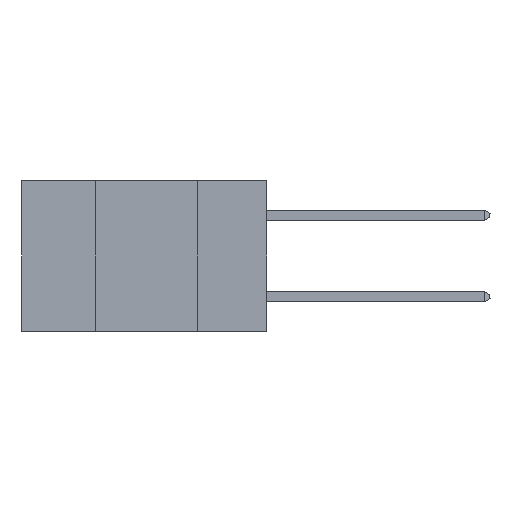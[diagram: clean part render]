
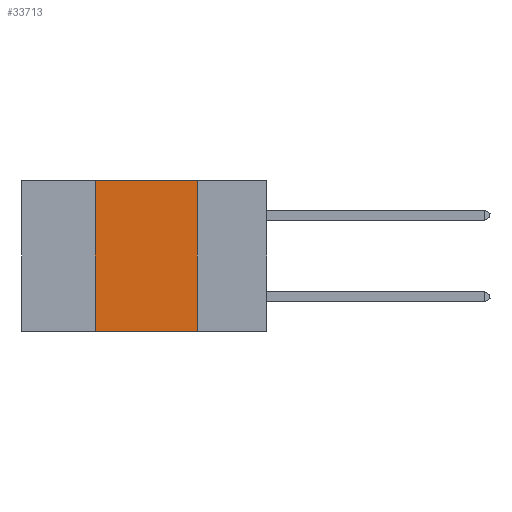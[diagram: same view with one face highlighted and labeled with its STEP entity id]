
A CAD part, left-side view. The second image highlights one B-rep face of the part: STEP entity #33713.
In plain terms, the highlighted planar face has unit normal (-1, 0, 0).
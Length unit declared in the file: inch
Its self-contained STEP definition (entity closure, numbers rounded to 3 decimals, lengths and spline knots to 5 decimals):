
#1861 = AXIS2_PLACEMENT_3D ( 'NONE', #5894, #24142, #1990 ) ;
#1990 = DIRECTION ( 'NONE',  ( 0., 0., -1. ) ) ;
#2196 = CARTESIAN_POINT ( 'NONE',  ( 0., 0.17, 0. ) ) ;
#4526 = VECTOR ( 'NONE', #17245, 39.37008 ) ;
#4668 = CARTESIAN_POINT ( 'NONE',  ( 0., 0.6, -0.37 ) ) ;
#4894 = EDGE_CURVE ( 'NONE', #17789, #32088, #27864, .T. ) ;
#5894 = CARTESIAN_POINT ( 'NONE',  ( 0., 0.6, 0. ) ) ;
#7902 = LINE ( 'NONE', #2196, #39862 ) ;
#8974 = ORIENTED_EDGE ( 'NONE', *, *, #31294, .F. ) ;
#9888 = DIRECTION ( 'NONE',  ( 0., 0., -1. ) ) ;
#9952 = FACE_OUTER_BOUND ( 'NONE', #28136, .T. ) ;
#10345 = ORIENTED_EDGE ( 'NONE', *, *, #4894, .T. ) ;
#12208 = DIRECTION ( 'NONE',  ( 0., -1., 0. ) ) ;
#13765 = LINE ( 'NONE', #30913, #31189 ) ;
#16289 = EDGE_CURVE ( 'NONE', #40742, #32088, #7902, .T. ) ;
#17113 = ORIENTED_EDGE ( 'NONE', *, *, #36325, .F. ) ;
#17245 = DIRECTION ( 'NONE',  ( 0., -1., 0. ) ) ;
#17789 = VERTEX_POINT ( 'NONE', #23036 ) ;
#19477 = CARTESIAN_POINT ( 'NONE',  ( 0., 0.17, 0. ) ) ;
#23036 = CARTESIAN_POINT ( 'NONE',  ( 0., 0.42, -0.37 ) ) ;
#24142 = DIRECTION ( 'NONE',  ( 1., 0., 0. ) ) ;
#24302 = PLANE ( 'NONE',  #1861 ) ;
#24711 = CARTESIAN_POINT ( 'NONE',  ( 0., 0.6, 0. ) ) ;
#27864 = LINE ( 'NONE', #4668, #38877 ) ;
#28136 = EDGE_LOOP ( 'NONE', ( #45336, #8974, #17113, #10345 ) ) ;
#30913 = CARTESIAN_POINT ( 'NONE',  ( 0., 0.42, 0. ) ) ;
#31189 = VECTOR ( 'NONE', #34618, 39.37008 ) ;
#31294 = EDGE_CURVE ( 'NONE', #34179, #40742, #47540, .T. ) ;
#32088 = VERTEX_POINT ( 'NONE', #44233 ) ;
#33713 = ADVANCED_FACE ( 'NONE', ( #9952 ), #24302, .F. ) ;
#34179 = VERTEX_POINT ( 'NONE', #41258 ) ;
#34618 = DIRECTION ( 'NONE',  ( 0., 0., 1. ) ) ;
#36325 = EDGE_CURVE ( 'NONE', #17789, #34179, #13765, .T. ) ;
#38877 = VECTOR ( 'NONE', #12208, 39.37008 ) ;
#39862 = VECTOR ( 'NONE', #9888, 39.37008 ) ;
#40742 = VERTEX_POINT ( 'NONE', #19477 ) ;
#41258 = CARTESIAN_POINT ( 'NONE',  ( 0., 0.42, 0. ) ) ;
#44233 = CARTESIAN_POINT ( 'NONE',  ( 0., 0.17, -0.37 ) ) ;
#45336 = ORIENTED_EDGE ( 'NONE', *, *, #16289, .F. ) ;
#47540 = LINE ( 'NONE', #24711, #4526 ) ;
